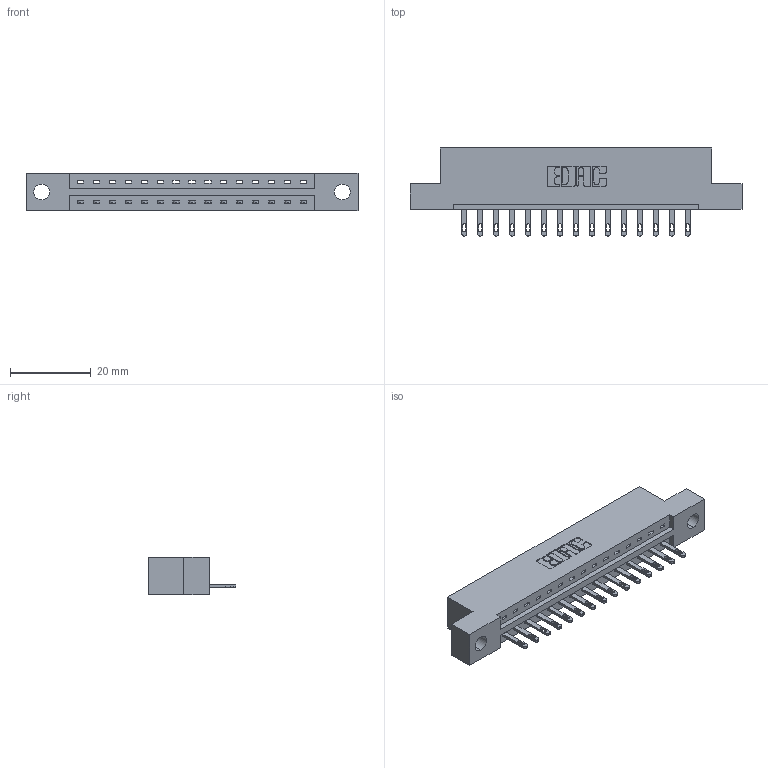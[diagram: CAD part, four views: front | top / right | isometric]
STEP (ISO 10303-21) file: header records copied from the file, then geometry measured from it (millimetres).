
FILE_DESCRIPTION (( 'STEP AP203' ), '1' );
FILE_NAME ('337-015-500-104.STEP', '2018-08-04T16:24:02', ( '' ), ( '' ), 'SwSTEP 2.0', 'SolidWorks 2016', '' );
FILE_SCHEMA (( 'CONFIG_CONTROL_DESIGN' ));
Length unit declared in the file: inch
Products named in the file (3): 345-292-001_345-293-100; 337-015-500-104; 337 Part_Flush Mounting Lugs - 0.156 Dia-TH
Assembly tree (16 placements, depth 2):
  337-015-500-104
    337 Part_Flush Mounting Lugs - 0.156 Dia-TH
    345-292-001_345-293-100  x15
Bounding box: 82.45 x 21.85 x 9.4 mm (x, y, z)
Volume: 8152.7 mm3; surface area: 8105 mm2
Topology: 16 solids, 16 shells, 984 faces, 3011 edges, 2006 vertices
Faces by surface type: plane 670, cylinder 314
Entity records: 14575 total; most frequent: CARTESIAN_POINT 2543, ORIENTED_EDGE 2494, DIRECTION 2197, EDGE_CURVE 1247, VECTOR 1115, LINE 1115, VERTEX_POINT 830, AXIS2_PLACEMENT_3D 541
